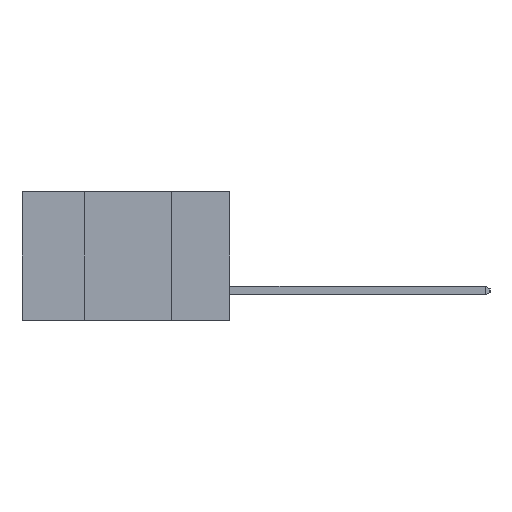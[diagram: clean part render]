
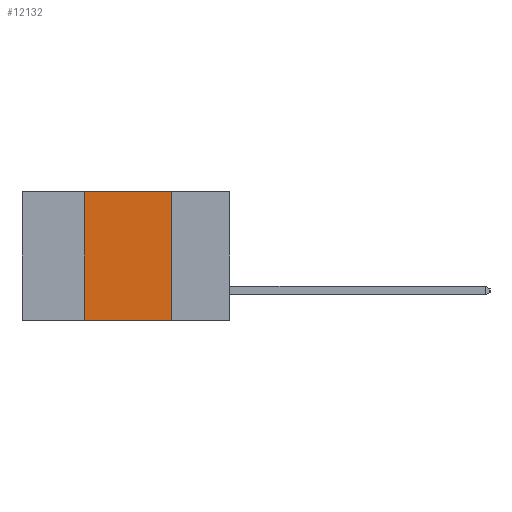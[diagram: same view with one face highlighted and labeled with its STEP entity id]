
A CAD part, left-side view. The second image highlights one B-rep face of the part: STEP entity #12132.
In plain terms, the highlighted planar face has unit normal (-1, 0, 0).
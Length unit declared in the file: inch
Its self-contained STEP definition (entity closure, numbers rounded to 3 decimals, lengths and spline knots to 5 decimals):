
#596 = FACE_OUTER_BOUND ( 'NONE', #7460, .T. ) ;
#809 = CARTESIAN_POINT ( 'NONE',  ( 0., 0.42, 0. ) ) ;
#814 = LINE ( 'NONE', #10062, #13518 ) ;
#1299 = VERTEX_POINT ( 'NONE', #809 ) ;
#1847 = LINE ( 'NONE', #12788, #8537 ) ;
#2305 = EDGE_CURVE ( 'NONE', #6612, #3196, #9268, .T. ) ;
#2798 = CARTESIAN_POINT ( 'NONE',  ( 0., 0.42, -0.37 ) ) ;
#2843 = EDGE_CURVE ( 'NONE', #13430, #3196, #5522, .T. ) ;
#3196 = VERTEX_POINT ( 'NONE', #6702 ) ;
#4830 = EDGE_CURVE ( 'NONE', #6612, #1299, #1847, .T. ) ;
#5086 = DIRECTION ( 'NONE',  ( 0., -1., 0. ) ) ;
#5522 = LINE ( 'NONE', #9915, #11705 ) ;
#6294 = CARTESIAN_POINT ( 'NONE',  ( 0., 0.6, 0. ) ) ;
#6516 = EDGE_CURVE ( 'NONE', #1299, #13430, #814, .T. ) ;
#6612 = VERTEX_POINT ( 'NONE', #2798 ) ;
#6702 = CARTESIAN_POINT ( 'NONE',  ( 0., 0.17, -0.37 ) ) ;
#7460 = EDGE_LOOP ( 'NONE', ( #11406, #12295, #13192, #13682 ) ) ;
#7565 = DIRECTION ( 'NONE',  ( 0., 0., -1. ) ) ;
#8537 = VECTOR ( 'NONE', #12551, 39.37008 ) ;
#9268 = LINE ( 'NONE', #13470, #9646 ) ;
#9646 = VECTOR ( 'NONE', #13520, 39.37008 ) ;
#9893 = DIRECTION ( 'NONE',  ( 0., 0., -1. ) ) ;
#9915 = CARTESIAN_POINT ( 'NONE',  ( 0., 0.17, -0.37 ) ) ;
#10062 = CARTESIAN_POINT ( 'NONE',  ( 0., 0.6, 0. ) ) ;
#11406 = ORIENTED_EDGE ( 'NONE', *, *, #2843, .F. ) ;
#11705 = VECTOR ( 'NONE', #9893, 39.37008 ) ;
#12132 = ADVANCED_FACE ( 'NONE', ( #596 ), #13542, .F. ) ;
#12295 = ORIENTED_EDGE ( 'NONE', *, *, #6516, .F. ) ;
#12551 = DIRECTION ( 'NONE',  ( 0., 0., 1. ) ) ;
#12788 = CARTESIAN_POINT ( 'NONE',  ( 0., 0.42, -0.37 ) ) ;
#13192 = ORIENTED_EDGE ( 'NONE', *, *, #4830, .F. ) ;
#13430 = VERTEX_POINT ( 'NONE', #13711 ) ;
#13470 = CARTESIAN_POINT ( 'NONE',  ( 0., 0.6, -0.37 ) ) ;
#13518 = VECTOR ( 'NONE', #5086, 39.37008 ) ;
#13520 = DIRECTION ( 'NONE',  ( 0., -1., 0. ) ) ;
#13542 = PLANE ( 'NONE',  #13971 ) ;
#13682 = ORIENTED_EDGE ( 'NONE', *, *, #2305, .T. ) ;
#13711 = CARTESIAN_POINT ( 'NONE',  ( 0., 0.17, 0. ) ) ;
#13971 = AXIS2_PLACEMENT_3D ( 'NONE', #6294, #14679, #7565 ) ;
#14679 = DIRECTION ( 'NONE',  ( 1., 0., 0. ) ) ;
